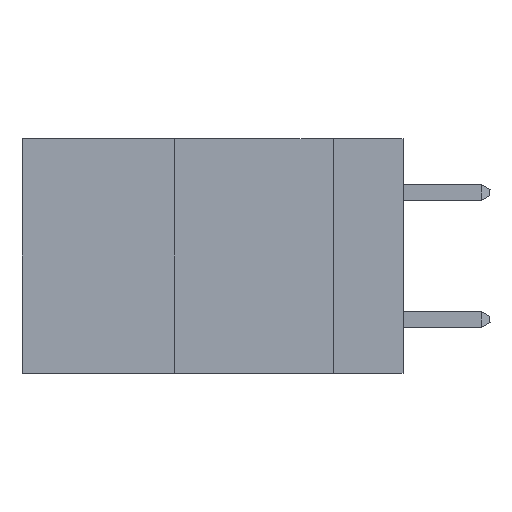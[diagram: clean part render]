
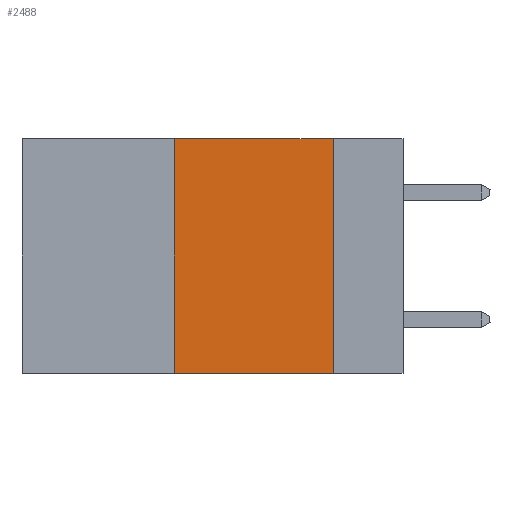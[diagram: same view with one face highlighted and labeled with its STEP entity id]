
A CAD part, left-side view. The second image highlights one B-rep face of the part: STEP entity #2488.
In plain terms, the highlighted planar face has unit normal (-1, 0, 0).
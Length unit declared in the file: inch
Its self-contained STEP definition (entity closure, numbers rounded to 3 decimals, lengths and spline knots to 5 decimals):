
#34 = ORIENTED_EDGE ( 'NONE', *, *, #620, .F. ) ;
#175 = CARTESIAN_POINT ( 'NONE',  ( 0., 0.36, 0. ) ) ;
#333 = DIRECTION ( 'NONE',  ( 0., -1., 0. ) ) ;
#620 = EDGE_CURVE ( 'NONE', #4205, #2239, #5664, .T. ) ;
#1286 = CARTESIAN_POINT ( 'NONE',  ( 0., 0.6, -0.37 ) ) ;
#1494 = DIRECTION ( 'NONE',  ( 1., 0., 0. ) ) ;
#1578 = LINE ( 'NONE', #5498, #5875 ) ;
#1614 = ORIENTED_EDGE ( 'NONE', *, *, #6404, .T. ) ;
#1850 = EDGE_LOOP ( 'NONE', ( #3504, #34, #2124, #1614 ) ) ;
#2124 = ORIENTED_EDGE ( 'NONE', *, *, #6141, .F. ) ;
#2134 = CARTESIAN_POINT ( 'NONE',  ( 0., 0.11, -0.37 ) ) ;
#2239 = VERTEX_POINT ( 'NONE', #3539 ) ;
#2488 = ADVANCED_FACE ( 'NONE', ( #5656 ), #7059, .F. ) ;
#3049 = VERTEX_POINT ( 'NONE', #2134 ) ;
#3064 = DIRECTION ( 'NONE',  ( 0., 0., -1. ) ) ;
#3342 = VECTOR ( 'NONE', #6943, 39.37008 ) ;
#3382 = DIRECTION ( 'NONE',  ( 0., 0., 1. ) ) ;
#3472 = CARTESIAN_POINT ( 'NONE',  ( 0., 0.6, 0. ) ) ;
#3504 = ORIENTED_EDGE ( 'NONE', *, *, #5675, .F. ) ;
#3539 = CARTESIAN_POINT ( 'NONE',  ( 0., 0.11, 0. ) ) ;
#3719 = VECTOR ( 'NONE', #3382, 39.37008 ) ;
#3770 = CARTESIAN_POINT ( 'NONE',  ( 0., 0.36, 0. ) ) ;
#3881 = CARTESIAN_POINT ( 'NONE',  ( 0., 0.6, 0. ) ) ;
#4205 = VERTEX_POINT ( 'NONE', #3770 ) ;
#5395 = VECTOR ( 'NONE', #333, 39.37008 ) ;
#5498 = CARTESIAN_POINT ( 'NONE',  ( 0., 0.11, 0. ) ) ;
#5656 = FACE_OUTER_BOUND ( 'NONE', #1850, .T. ) ;
#5664 = LINE ( 'NONE', #3881, #5395 ) ;
#5675 = EDGE_CURVE ( 'NONE', #2239, #3049, #1578, .T. ) ;
#5875 = VECTOR ( 'NONE', #3064, 39.37008 ) ;
#6141 = EDGE_CURVE ( 'NONE', #7921, #4205, #8262, .T. ) ;
#6404 = EDGE_CURVE ( 'NONE', #7921, #3049, #7389, .T. ) ;
#6537 = CARTESIAN_POINT ( 'NONE',  ( 0., 0.36, -0.37 ) ) ;
#6943 = DIRECTION ( 'NONE',  ( 0., -1., 0. ) ) ;
#7059 = PLANE ( 'NONE',  #7241 ) ;
#7241 = AXIS2_PLACEMENT_3D ( 'NONE', #3472, #1494, #9034 ) ;
#7389 = LINE ( 'NONE', #1286, #3342 ) ;
#7921 = VERTEX_POINT ( 'NONE', #6537 ) ;
#8262 = LINE ( 'NONE', #175, #3719 ) ;
#9034 = DIRECTION ( 'NONE',  ( 0., 0., -1. ) ) ;
